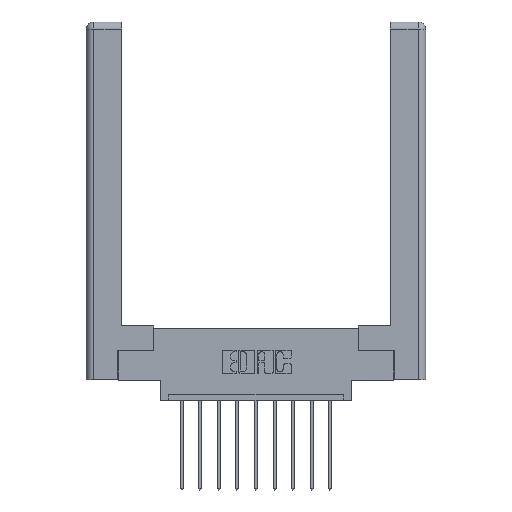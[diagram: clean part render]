
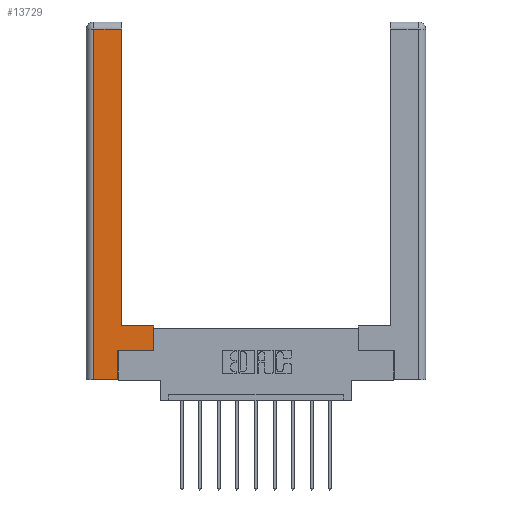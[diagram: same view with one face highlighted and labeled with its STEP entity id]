
A CAD part, top view. The second image highlights one B-rep face of the part: STEP entity #13729.
In plain terms, the highlighted planar face has unit normal (0, 0, 1).
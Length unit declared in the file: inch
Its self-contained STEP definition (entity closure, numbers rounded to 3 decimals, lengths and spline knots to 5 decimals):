
#400 = DIRECTION ( 'NONE',  ( 0., 1., 0. ) ) ;
#406 = DIRECTION ( 'NONE',  ( -1., 0., 0. ) ) ;
#497 = VERTEX_POINT ( 'NONE', #7139 ) ;
#885 = EDGE_CURVE ( 'NONE', #497, #1725, #4191, .T. ) ;
#961 = CARTESIAN_POINT ( 'NONE',  ( 0.265, 0., 0. ) ) ;
#1299 = LINE ( 'NONE', #6168, #1638 ) ;
#1472 = VECTOR ( 'NONE', #12542, 39.37008 ) ;
#1638 = VECTOR ( 'NONE', #4131, 39.37008 ) ;
#1680 = VECTOR ( 'NONE', #2907, 39.37008 ) ;
#1725 = VERTEX_POINT ( 'NONE', #13241 ) ;
#1998 = ORIENTED_EDGE ( 'NONE', *, *, #9588, .T. ) ;
#2223 = ORIENTED_EDGE ( 'NONE', *, *, #10236, .T. ) ;
#2354 = LINE ( 'NONE', #6452, #7767 ) ;
#2497 = DIRECTION ( 'NONE',  ( 0., 1., 0. ) ) ;
#2539 = EDGE_CURVE ( 'NONE', #13217, #3432, #1299, .T. ) ;
#2907 = DIRECTION ( 'NONE',  ( 0., 1., 0. ) ) ;
#3048 = VECTOR ( 'NONE', #12917, 39.37008 ) ;
#3148 = VERTEX_POINT ( 'NONE', #11986 ) ;
#3432 = VERTEX_POINT ( 'NONE', #8852 ) ;
#3551 = VERTEX_POINT ( 'NONE', #4783 ) ;
#3704 = LINE ( 'NONE', #13307, #10186 ) ;
#3946 = EDGE_CURVE ( 'NONE', #3551, #3148, #3704, .T. ) ;
#4131 = DIRECTION ( 'NONE',  ( -1., 0., 0. ) ) ;
#4191 = LINE ( 'NONE', #12136, #3048 ) ;
#4250 = CARTESIAN_POINT ( 'NONE',  ( 0.295, 2.94, 0. ) ) ;
#4783 = CARTESIAN_POINT ( 'NONE',  ( 0.565, 0.45, 0. ) ) ;
#5088 = DIRECTION ( 'NONE',  ( -1., 0., 0. ) ) ;
#5578 = EDGE_CURVE ( 'NONE', #3148, #13217, #9531, .T. ) ;
#5984 = ORIENTED_EDGE ( 'NONE', *, *, #12340, .T. ) ;
#6168 = CARTESIAN_POINT ( 'NONE',  ( 0.0615, 2.94, 0. ) ) ;
#6201 = FACE_OUTER_BOUND ( 'NONE', #8646, .T. ) ;
#6452 = CARTESIAN_POINT ( 'NONE',  ( 0.0615, 0., 0. ) ) ;
#6828 = CARTESIAN_POINT ( 'NONE',  ( 0.0615, 0., 0. ) ) ;
#6942 = ORIENTED_EDGE ( 'NONE', *, *, #3946, .T. ) ;
#7139 = CARTESIAN_POINT ( 'NONE',  ( 0.265, 0.245, 0. ) ) ;
#7183 = EDGE_CURVE ( 'NONE', #7771, #497, #11930, .T. ) ;
#7620 = VECTOR ( 'NONE', #2497, 39.37008 ) ;
#7767 = VECTOR ( 'NONE', #11717, 39.37008 ) ;
#7771 = VERTEX_POINT ( 'NONE', #961 ) ;
#8646 = EDGE_LOOP ( 'NONE', ( #13258, #11560, #2223, #5984, #11547, #13249, #1998, #6942 ) ) ;
#8829 = VECTOR ( 'NONE', #400, 39.37008 ) ;
#8852 = CARTESIAN_POINT ( 'NONE',  ( 0.0615, 2.94, 0. ) ) ;
#9236 = CARTESIAN_POINT ( 'NONE',  ( 0.265, 0.245, 0. ) ) ;
#9462 = CARTESIAN_POINT ( 'NONE',  ( 0., 0., 0. ) ) ;
#9531 = LINE ( 'NONE', #11994, #8829 ) ;
#9588 = EDGE_CURVE ( 'NONE', #1725, #3551, #13639, .T. ) ;
#9864 = AXIS2_PLACEMENT_3D ( 'NONE', #9462, #10365, #5088 ) ;
#10186 = VECTOR ( 'NONE', #406, 39.37008 ) ;
#10236 = EDGE_CURVE ( 'NONE', #3432, #11783, #2354, .T. ) ;
#10240 = LINE ( 'NONE', #12356, #1472 ) ;
#10365 = DIRECTION ( 'NONE',  ( 0., 0., -1. ) ) ;
#10406 = PLANE ( 'NONE',  #9864 ) ;
#11547 = ORIENTED_EDGE ( 'NONE', *, *, #7183, .T. ) ;
#11560 = ORIENTED_EDGE ( 'NONE', *, *, #2539, .T. ) ;
#11717 = DIRECTION ( 'NONE',  ( 0., -1., 0. ) ) ;
#11783 = VERTEX_POINT ( 'NONE', #6828 ) ;
#11930 = LINE ( 'NONE', #9236, #1680 ) ;
#11986 = CARTESIAN_POINT ( 'NONE',  ( 0.295, 0.45, 0. ) ) ;
#11994 = CARTESIAN_POINT ( 'NONE',  ( 0.295, 3., 0. ) ) ;
#12136 = CARTESIAN_POINT ( 'NONE',  ( 0.565, 0.245, 0. ) ) ;
#12340 = EDGE_CURVE ( 'NONE', #11783, #7771, #10240, .T. ) ;
#12356 = CARTESIAN_POINT ( 'NONE',  ( 0.265, 0., 0. ) ) ;
#12542 = DIRECTION ( 'NONE',  ( 1., 0., 0. ) ) ;
#12917 = DIRECTION ( 'NONE',  ( 1., 0., 0. ) ) ;
#12950 = CARTESIAN_POINT ( 'NONE',  ( 0.565, 0.45, 0. ) ) ;
#13217 = VERTEX_POINT ( 'NONE', #4250 ) ;
#13241 = CARTESIAN_POINT ( 'NONE',  ( 0.565, 0.245, 0. ) ) ;
#13249 = ORIENTED_EDGE ( 'NONE', *, *, #885, .T. ) ;
#13258 = ORIENTED_EDGE ( 'NONE', *, *, #5578, .T. ) ;
#13307 = CARTESIAN_POINT ( 'NONE',  ( 0.295, 0.45, 0. ) ) ;
#13639 = LINE ( 'NONE', #12950, #7620 ) ;
#13729 = ADVANCED_FACE ( 'NONE', ( #6201 ), #10406, .F. ) ;
